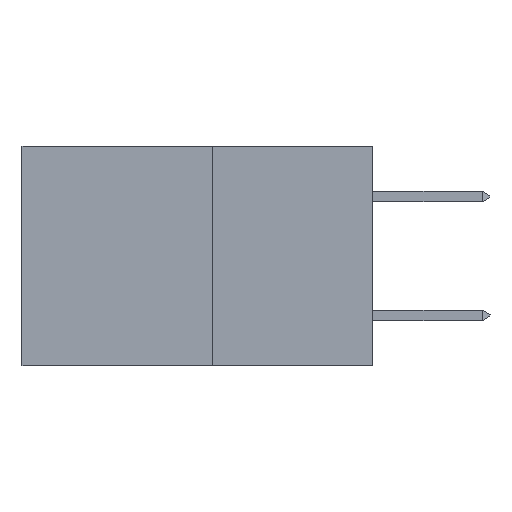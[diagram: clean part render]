
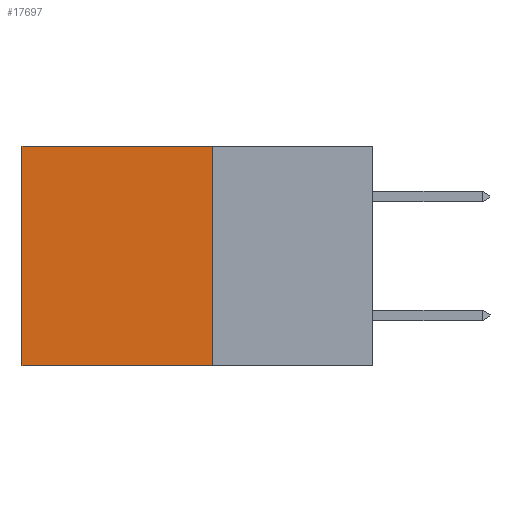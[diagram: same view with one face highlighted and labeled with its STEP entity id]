
A CAD part, left-side view. The second image highlights one B-rep face of the part: STEP entity #17697.
In plain terms, the highlighted planar face has unit normal (-1, 0, 0).
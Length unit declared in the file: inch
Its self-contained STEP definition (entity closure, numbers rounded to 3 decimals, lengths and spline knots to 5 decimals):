
#654 = DIRECTION ( 'NONE',  ( 0., 0., -1. ) ) ;
#1395 = LINE ( 'NONE', #15916, #9617 ) ;
#1442 = DIRECTION ( 'NONE',  ( 0., 1., 0. ) ) ;
#1975 = VERTEX_POINT ( 'NONE', #19926 ) ;
#2556 = ORIENTED_EDGE ( 'NONE', *, *, #16717, .T. ) ;
#2954 = CARTESIAN_POINT ( 'NONE',  ( 0.277, 0.27, -0.37 ) ) ;
#3487 = LINE ( 'NONE', #10654, #15710 ) ;
#3710 = CARTESIAN_POINT ( 'NONE',  ( 0.277, 0.27, -0.37 ) ) ;
#5229 = ORIENTED_EDGE ( 'NONE', *, *, #16136, .F. ) ;
#5554 = VECTOR ( 'NONE', #1442, 39.37008 ) ;
#6731 = VECTOR ( 'NONE', #7862, 39.37008 ) ;
#6872 = AXIS2_PLACEMENT_3D ( 'NONE', #16665, #10517, #654 ) ;
#7589 = VERTEX_POINT ( 'NONE', #9799 ) ;
#7862 = DIRECTION ( 'NONE',  ( 0., 1., 0. ) ) ;
#8849 = ORIENTED_EDGE ( 'NONE', *, *, #15296, .F. ) ;
#9454 = VERTEX_POINT ( 'NONE', #18416 ) ;
#9617 = VECTOR ( 'NONE', #17393, 39.37008 ) ;
#9799 = CARTESIAN_POINT ( 'NONE',  ( 0.277, 0.59, 0. ) ) ;
#10517 = DIRECTION ( 'NONE',  ( 1., 0., 0. ) ) ;
#10654 = CARTESIAN_POINT ( 'NONE',  ( 0.277, 0.27, -0.37 ) ) ;
#11060 = VERTEX_POINT ( 'NONE', #3710 ) ;
#11539 = LINE ( 'NONE', #2954, #6731 ) ;
#12240 = DIRECTION ( 'NONE',  ( 0., 0., -1. ) ) ;
#12924 = ORIENTED_EDGE ( 'NONE', *, *, #14248, .T. ) ;
#14074 = LINE ( 'NONE', #20178, #5554 ) ;
#14248 = EDGE_CURVE ( 'NONE', #1975, #7589, #14074, .T. ) ;
#15178 = PLANE ( 'NONE',  #6872 ) ;
#15296 = EDGE_CURVE ( 'NONE', #1975, #11060, #3487, .T. ) ;
#15710 = VECTOR ( 'NONE', #12240, 39.37008 ) ;
#15916 = CARTESIAN_POINT ( 'NONE',  ( 0.277, 0.59, -0.37 ) ) ;
#16136 = EDGE_CURVE ( 'NONE', #11060, #9454, #11539, .T. ) ;
#16665 = CARTESIAN_POINT ( 'NONE',  ( 0.277, 0.27, -0.37 ) ) ;
#16717 = EDGE_CURVE ( 'NONE', #7589, #9454, #1395, .T. ) ;
#17393 = DIRECTION ( 'NONE',  ( 0., 0., -1. ) ) ;
#17697 = ADVANCED_FACE ( 'NONE', ( #18423 ), #15178, .F. ) ;
#18416 = CARTESIAN_POINT ( 'NONE',  ( 0.277, 0.59, -0.37 ) ) ;
#18423 = FACE_OUTER_BOUND ( 'NONE', #18888, .T. ) ;
#18888 = EDGE_LOOP ( 'NONE', ( #2556, #5229, #8849, #12924 ) ) ;
#19926 = CARTESIAN_POINT ( 'NONE',  ( 0.277, 0.27, 0. ) ) ;
#20178 = CARTESIAN_POINT ( 'NONE',  ( 0.277, 0.27, 0. ) ) ;
